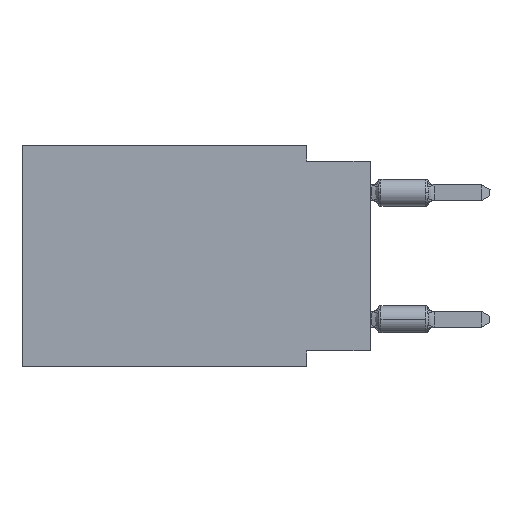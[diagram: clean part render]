
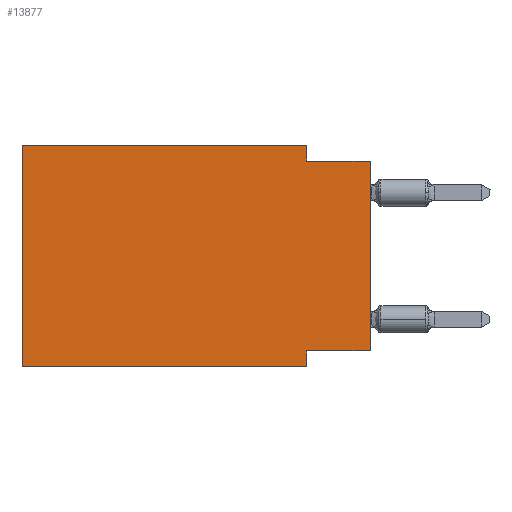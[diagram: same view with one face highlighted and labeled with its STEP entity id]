
A CAD part, left-side view. The second image highlights one B-rep face of the part: STEP entity #13877.
In plain terms, the highlighted planar face has unit normal (-1, 0, 0).
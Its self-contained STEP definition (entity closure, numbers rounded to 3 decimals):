
#1464 = EDGE_CURVE ( 'NONE', #1559, #23526, #35466, .T. ) ;
#1559 = VERTEX_POINT ( 'NONE', #51747 ) ;
#2755 = LINE ( 'NONE', #44260, #44298 ) ;
#2977 = LINE ( 'NONE', #7404, #40337 ) ;
#3023 = DIRECTION ( 'NONE',  ( 0., -1., 0. ) ) ;
#3232 = VECTOR ( 'NONE', #27296, 1000. ) ;
#3251 = DIRECTION ( 'NONE',  ( 0., 0., 1. ) ) ;
#4148 = VERTEX_POINT ( 'NONE', #40403 ) ;
#4921 = DIRECTION ( 'NONE',  ( 0., 1., 0. ) ) ;
#7313 = ORIENTED_EDGE ( 'NONE', *, *, #11419, .F. ) ;
#7404 = CARTESIAN_POINT ( 'NONE',  ( 0., 13.97, 0. ) ) ;
#7877 = VECTOR ( 'NONE', #12946, 1000. ) ;
#8154 = VERTEX_POINT ( 'NONE', #16522 ) ;
#8606 = CARTESIAN_POINT ( 'NONE',  ( 0., 2.54, -8.255 ) ) ;
#9908 = CARTESIAN_POINT ( 'NONE',  ( 0., 13.97, -8.89 ) ) ;
#10053 = CARTESIAN_POINT ( 'NONE',  ( 0., 2.54, 0. ) ) ;
#10715 = CARTESIAN_POINT ( 'NONE',  ( 0., 13.97, -8.89 ) ) ;
#11077 = FACE_OUTER_BOUND ( 'NONE', #27660, .T. ) ;
#11343 = EDGE_CURVE ( 'NONE', #39501, #17163, #28391, .T. ) ;
#11419 = EDGE_CURVE ( 'NONE', #51152, #17163, #44979, .T. ) ;
#12946 = DIRECTION ( 'NONE',  ( 0., -1., 0. ) ) ;
#13877 = ADVANCED_FACE ( 'NONE', ( #11077 ), #39846, .F. ) ;
#16332 = EDGE_CURVE ( 'NONE', #4148, #23526, #2755, .T. ) ;
#16522 = CARTESIAN_POINT ( 'NONE',  ( 0., 13.97, 0. ) ) ;
#17163 = VERTEX_POINT ( 'NONE', #32166 ) ;
#17667 = CARTESIAN_POINT ( 'NONE',  ( 0., 0., -8.255 ) ) ;
#17805 = ORIENTED_EDGE ( 'NONE', *, *, #40670, .F. ) ;
#19099 = CARTESIAN_POINT ( 'NONE',  ( 0., 13.97, 0. ) ) ;
#22696 = VECTOR ( 'NONE', #44019, 1000. ) ;
#22939 = ORIENTED_EDGE ( 'NONE', *, *, #16332, .F. ) ;
#23526 = VERTEX_POINT ( 'NONE', #48997 ) ;
#23545 = VECTOR ( 'NONE', #53519, 1000. ) ;
#26109 = DIRECTION ( 'NONE',  ( 0., 0., -1. ) ) ;
#26924 = ORIENTED_EDGE ( 'NONE', *, *, #11343, .T. ) ;
#27125 = DIRECTION ( 'NONE',  ( 1., 0., 0. ) ) ;
#27296 = DIRECTION ( 'NONE',  ( 0., -1., 0. ) ) ;
#27660 = EDGE_LOOP ( 'NONE', ( #37920, #22939, #34201, #39659, #50315, #26924, #7313, #17805 ) ) ;
#28391 = LINE ( 'NONE', #10715, #3232 ) ;
#28844 = EDGE_CURVE ( 'NONE', #39501, #8154, #2977, .T. ) ;
#30657 = LINE ( 'NONE', #17667, #53676 ) ;
#31576 = CARTESIAN_POINT ( 'NONE',  ( 0., 0., 0. ) ) ;
#32166 = CARTESIAN_POINT ( 'NONE',  ( 0., 2.54, -8.89 ) ) ;
#34201 = ORIENTED_EDGE ( 'NONE', *, *, #54028, .F. ) ;
#34240 = CARTESIAN_POINT ( 'NONE',  ( 0., 13.97, 0. ) ) ;
#35466 = LINE ( 'NONE', #31576, #22696 ) ;
#36690 = CARTESIAN_POINT ( 'NONE',  ( 0., 2.54, -8.89 ) ) ;
#37920 = ORIENTED_EDGE ( 'NONE', *, *, #1464, .T. ) ;
#38027 = AXIS2_PLACEMENT_3D ( 'NONE', #19099, #27125, #53348 ) ;
#39501 = VERTEX_POINT ( 'NONE', #9908 ) ;
#39659 = ORIENTED_EDGE ( 'NONE', *, *, #41938, .F. ) ;
#39846 = PLANE ( 'NONE',  #38027 ) ;
#40337 = VECTOR ( 'NONE', #3251, 1000. ) ;
#40354 = VERTEX_POINT ( 'NONE', #10053 ) ;
#40403 = CARTESIAN_POINT ( 'NONE',  ( 0., 2.54, -0.635 ) ) ;
#40670 = EDGE_CURVE ( 'NONE', #1559, #51152, #30657, .T. ) ;
#41938 = EDGE_CURVE ( 'NONE', #8154, #40354, #46661, .T. ) ;
#43856 = VECTOR ( 'NONE', #26109, 1000. ) ;
#44019 = DIRECTION ( 'NONE',  ( 0., 0., 1. ) ) ;
#44066 = CARTESIAN_POINT ( 'NONE',  ( 0., 2.54, 0. ) ) ;
#44260 = CARTESIAN_POINT ( 'NONE',  ( 0., 0., -0.635 ) ) ;
#44298 = VECTOR ( 'NONE', #3023, 1000. ) ;
#44979 = LINE ( 'NONE', #36690, #23545 ) ;
#46661 = LINE ( 'NONE', #34240, #7877 ) ;
#47112 = LINE ( 'NONE', #44066, #43856 ) ;
#48997 = CARTESIAN_POINT ( 'NONE',  ( 0., 0., -0.635 ) ) ;
#50315 = ORIENTED_EDGE ( 'NONE', *, *, #28844, .F. ) ;
#51152 = VERTEX_POINT ( 'NONE', #8606 ) ;
#51747 = CARTESIAN_POINT ( 'NONE',  ( 0., 0., -8.255 ) ) ;
#53348 = DIRECTION ( 'NONE',  ( 0., 0., -1. ) ) ;
#53519 = DIRECTION ( 'NONE',  ( 0., 0., -1. ) ) ;
#53676 = VECTOR ( 'NONE', #4921, 1000. ) ;
#54028 = EDGE_CURVE ( 'NONE', #40354, #4148, #47112, .T. ) ;
